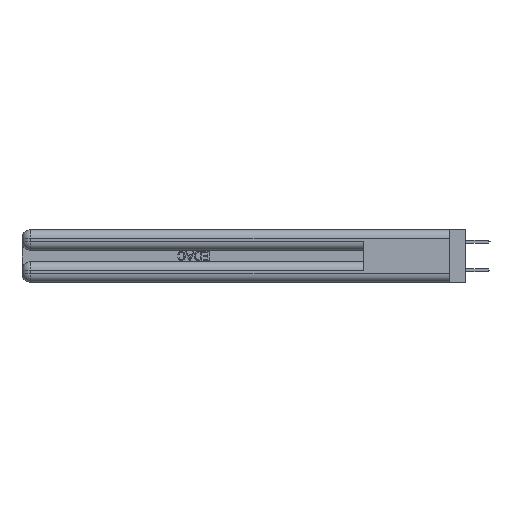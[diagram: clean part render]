
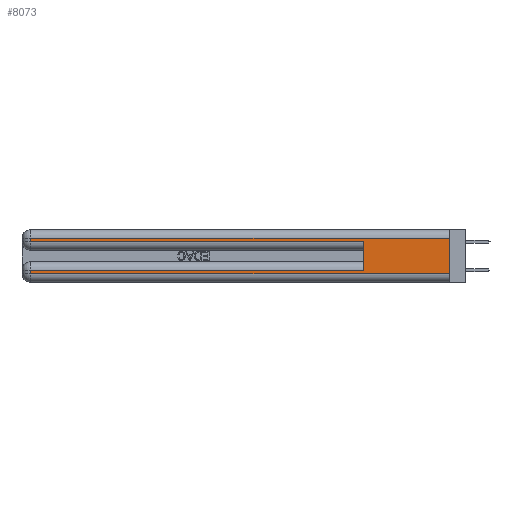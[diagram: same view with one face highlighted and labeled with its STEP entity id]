
A CAD part, left-side view. The second image highlights one B-rep face of the part: STEP entity #8073.
In plain terms, the highlighted planar face has unit normal (-1, 0, 0).
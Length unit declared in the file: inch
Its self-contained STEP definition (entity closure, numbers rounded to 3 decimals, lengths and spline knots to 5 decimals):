
#558 = ORIENTED_EDGE ( 'NONE', *, *, #35348, .F. ) ;
#681 = CARTESIAN_POINT ( 'NONE',  ( 0., 0., 0.085 ) ) ;
#979 = VECTOR ( 'NONE', #27019, 39.37008 ) ;
#987 = ORIENTED_EDGE ( 'NONE', *, *, #35579, .T. ) ;
#1310 = DIRECTION ( 'NONE',  ( 0., 0., -1. ) ) ;
#1471 = ORIENTED_EDGE ( 'NONE', *, *, #10549, .T. ) ;
#1690 = EDGE_LOOP ( 'NONE', ( #558, #987, #1471, #2485, #2783, #2862, #6769, #7306 ) ) ;
#2485 = ORIENTED_EDGE ( 'NONE', *, *, #27015, .T. ) ;
#2783 = ORIENTED_EDGE ( 'NONE', *, *, #25461, .F. ) ;
#2804 = VECTOR ( 'NONE', #20744, 39.37008 ) ;
#2862 = ORIENTED_EDGE ( 'NONE', *, *, #31883, .T. ) ;
#3277 = CARTESIAN_POINT ( 'NONE',  ( 0., 2.94, 0.37 ) ) ;
#3284 = CARTESIAN_POINT ( 'NONE',  ( 0., 0.6, 0.145 ) ) ;
#3358 = PLANE ( 'NONE',  #7867 ) ;
#3538 = CARTESIAN_POINT ( 'NONE',  ( 0., 2.94, 0.085 ) ) ;
#4181 = VECTOR ( 'NONE', #34268, 39.37008 ) ;
#4224 = LINE ( 'NONE', #681, #20923 ) ;
#5104 = LINE ( 'NONE', #25332, #4181 ) ;
#5506 = CARTESIAN_POINT ( 'NONE',  ( 0., 2.94, 0.285 ) ) ;
#6362 = DIRECTION ( 'NONE',  ( 1., 0., 0. ) ) ;
#6769 = ORIENTED_EDGE ( 'NONE', *, *, #17987, .T. ) ;
#7306 = ORIENTED_EDGE ( 'NONE', *, *, #22704, .T. ) ;
#7391 = DIRECTION ( 'NONE',  ( 0., 1., 0. ) ) ;
#7615 = VERTEX_POINT ( 'NONE', #33572 ) ;
#7867 = AXIS2_PLACEMENT_3D ( 'NONE', #21138, #6362, #27089 ) ;
#8073 = ADVANCED_FACE ( 'NONE', ( #35275 ), #3358, .F. ) ;
#8967 = LINE ( 'NONE', #3284, #979 ) ;
#9334 = LINE ( 'NONE', #3277, #24131 ) ;
#9972 = VECTOR ( 'NONE', #27087, 39.37008 ) ;
#10549 = EDGE_CURVE ( 'NONE', #25389, #30017, #29167, .T. ) ;
#13130 = CARTESIAN_POINT ( 'NONE',  ( 0., 0.6, 0.085 ) ) ;
#15173 = CARTESIAN_POINT ( 'NONE',  ( 0., 0., 0.37 ) ) ;
#17987 = EDGE_CURVE ( 'NONE', #36611, #30519, #9334, .T. ) ;
#18278 = LINE ( 'NONE', #25100, #19203 ) ;
#19203 = VECTOR ( 'NONE', #7391, 39.37008 ) ;
#19517 = LINE ( 'NONE', #35477, #2804 ) ;
#19661 = VERTEX_POINT ( 'NONE', #29176 ) ;
#20744 = DIRECTION ( 'NONE',  ( 0., -1., 0. ) ) ;
#20923 = VECTOR ( 'NONE', #21518, 39.37008 ) ;
#21138 = CARTESIAN_POINT ( 'NONE',  ( 0., 0., 0.37 ) ) ;
#21287 = VECTOR ( 'NONE', #1310, 39.37008 ) ;
#21518 = DIRECTION ( 'NONE',  ( 0., 1., 0. ) ) ;
#22127 = CARTESIAN_POINT ( 'NONE',  ( 0., 2.94, 0.37 ) ) ;
#22573 = CARTESIAN_POINT ( 'NONE',  ( 0., 2.94, 0.06 ) ) ;
#22704 = EDGE_CURVE ( 'NONE', #30519, #35722, #19517, .T. ) ;
#24131 = VECTOR ( 'NONE', #27012, 39.37008 ) ;
#25100 = CARTESIAN_POINT ( 'NONE',  ( 0., 0., 0.31 ) ) ;
#25332 = CARTESIAN_POINT ( 'NONE',  ( 0., 0., 0.285 ) ) ;
#25389 = VERTEX_POINT ( 'NONE', #35548 ) ;
#25461 = EDGE_CURVE ( 'NONE', #33186, #7615, #8967, .T. ) ;
#25737 = CARTESIAN_POINT ( 'NONE',  ( 0., 0., 0.06 ) ) ;
#27012 = DIRECTION ( 'NONE',  ( 0., 0., -1. ) ) ;
#27015 = EDGE_CURVE ( 'NONE', #30017, #7615, #5104, .T. ) ;
#27019 = DIRECTION ( 'NONE',  ( 0., 0., 1. ) ) ;
#27087 = DIRECTION ( 'NONE',  ( 0., 0., -1. ) ) ;
#27089 = DIRECTION ( 'NONE',  ( 0., 0., -1. ) ) ;
#29167 = LINE ( 'NONE', #22127, #21287 ) ;
#29176 = CARTESIAN_POINT ( 'NONE',  ( 0., 0., 0.31 ) ) ;
#30017 = VERTEX_POINT ( 'NONE', #5506 ) ;
#30519 = VERTEX_POINT ( 'NONE', #22573 ) ;
#31883 = EDGE_CURVE ( 'NONE', #33186, #36611, #4224, .T. ) ;
#33186 = VERTEX_POINT ( 'NONE', #13130 ) ;
#33572 = CARTESIAN_POINT ( 'NONE',  ( 0., 0.6, 0.285 ) ) ;
#34268 = DIRECTION ( 'NONE',  ( 0., -1., 0. ) ) ;
#34504 = LINE ( 'NONE', #15173, #9972 ) ;
#35275 = FACE_OUTER_BOUND ( 'NONE', #1690, .T. ) ;
#35348 = EDGE_CURVE ( 'NONE', #19661, #35722, #34504, .T. ) ;
#35477 = CARTESIAN_POINT ( 'NONE',  ( 0., 0., 0.06 ) ) ;
#35548 = CARTESIAN_POINT ( 'NONE',  ( 0., 2.94, 0.31 ) ) ;
#35579 = EDGE_CURVE ( 'NONE', #19661, #25389, #18278, .T. ) ;
#35722 = VERTEX_POINT ( 'NONE', #25737 ) ;
#36611 = VERTEX_POINT ( 'NONE', #3538 ) ;
